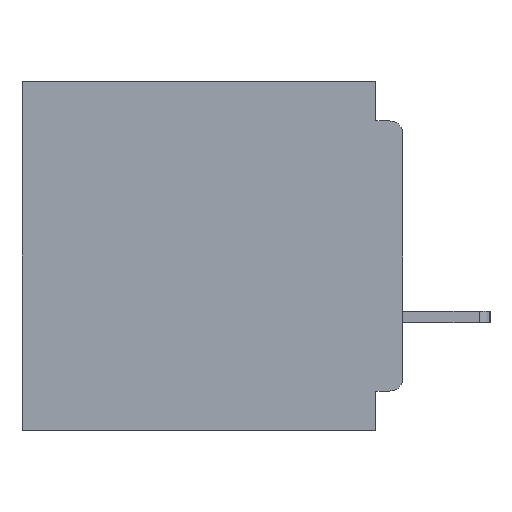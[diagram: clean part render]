
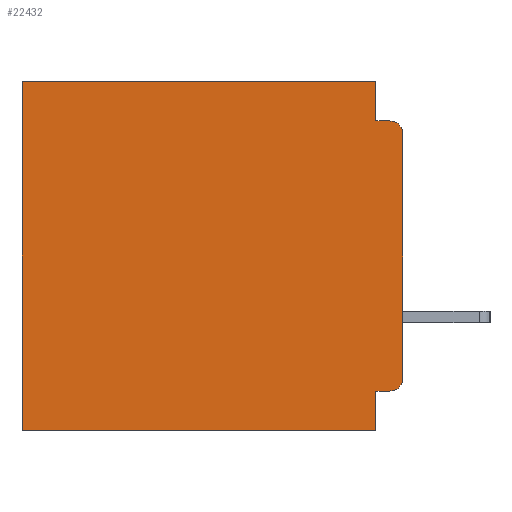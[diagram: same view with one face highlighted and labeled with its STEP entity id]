
A CAD part, left-side view. The second image highlights one B-rep face of the part: STEP entity #22432.
In plain terms, the highlighted planar face has unit normal (-1, 0, 0).
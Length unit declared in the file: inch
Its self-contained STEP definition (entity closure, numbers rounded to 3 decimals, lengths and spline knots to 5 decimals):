
#169 = ORIENTED_EDGE ( 'NONE', *, *, #23646, .F. ) ;
#470 = EDGE_LOOP ( 'NONE', ( #30593, #10990, #30169, #3765, #36550, #21946, #169, #10608, #33827, #23842 ) ) ;
#1314 = CARTESIAN_POINT ( 'NONE',  ( 0.3, 0.437, -0.4 ) ) ;
#1453 = VECTOR ( 'NONE', #3427, 39.37008 ) ;
#2436 = LINE ( 'NONE', #28248, #32483 ) ;
#2808 = DIRECTION ( 'NONE',  ( -1., 0., 0. ) ) ;
#3421 = VERTEX_POINT ( 'NONE', #35032 ) ;
#3427 = DIRECTION ( 'NONE',  ( 0., 0., -1. ) ) ;
#3627 = VERTEX_POINT ( 'NONE', #26118 ) ;
#3765 = ORIENTED_EDGE ( 'NONE', *, *, #23575, .F. ) ;
#4363 = VERTEX_POINT ( 'NONE', #7666 ) ;
#4952 = VERTEX_POINT ( 'NONE', #22074 ) ;
#4992 = DIRECTION ( 'NONE',  ( 0., 0., -1. ) ) ;
#5942 = DIRECTION ( 'NONE',  ( 0., 0., -1. ) ) ;
#5996 = DIRECTION ( 'NONE',  ( 0., 1., 0. ) ) ;
#6307 = VECTOR ( 'NONE', #5942, 39.37008 ) ;
#6898 = VERTEX_POINT ( 'NONE', #21006 ) ;
#7435 = EDGE_CURVE ( 'NONE', #3421, #3627, #36376, .T. ) ;
#7666 = CARTESIAN_POINT ( 'NONE',  ( 0.3, 0.031, -0.4 ) ) ;
#8458 = CIRCLE ( 'NONE', #8766, 0.015 ) ;
#8729 = CARTESIAN_POINT ( 'NONE',  ( 0.3, 0., -0.4 ) ) ;
#8766 = AXIS2_PLACEMENT_3D ( 'NONE', #20181, #2808, #23174 ) ;
#10187 = EDGE_CURVE ( 'NONE', #25279, #13175, #31366, .T. ) ;
#10572 = CARTESIAN_POINT ( 'NONE',  ( 0.3, 0.437, 0. ) ) ;
#10608 = ORIENTED_EDGE ( 'NONE', *, *, #18930, .F. ) ;
#10990 = ORIENTED_EDGE ( 'NONE', *, *, #14570, .T. ) ;
#11297 = CARTESIAN_POINT ( 'NONE',  ( 0.3, 0.031, -0.045 ) ) ;
#11483 = VECTOR ( 'NONE', #22999, 39.37008 ) ;
#11809 = DIRECTION ( 'NONE',  ( 0., 1., 0. ) ) ;
#12071 = EDGE_CURVE ( 'NONE', #3421, #16164, #8458, .T. ) ;
#12117 = DIRECTION ( 'NONE',  ( 1., 0., 0. ) ) ;
#13175 = VERTEX_POINT ( 'NONE', #1314 ) ;
#13344 = EDGE_CURVE ( 'NONE', #25405, #4952, #2436, .T. ) ;
#14570 = EDGE_CURVE ( 'NONE', #19447, #4952, #28294, .T. ) ;
#14644 = AXIS2_PLACEMENT_3D ( 'NONE', #17168, #37584, #20077 ) ;
#15597 = VECTOR ( 'NONE', #31936, 39.37008 ) ;
#15735 = AXIS2_PLACEMENT_3D ( 'NONE', #29598, #12117, #32507 ) ;
#16164 = VERTEX_POINT ( 'NONE', #19823 ) ;
#16492 = LINE ( 'NONE', #34873, #15597 ) ;
#16630 = DIRECTION ( 'NONE',  ( 0., -1., 0. ) ) ;
#17168 = CARTESIAN_POINT ( 'NONE',  ( 0.3, 0.015, -0.06 ) ) ;
#17323 = CARTESIAN_POINT ( 'NONE',  ( 0.3, 0., -0.06 ) ) ;
#18930 = EDGE_CURVE ( 'NONE', #3627, #4363, #31458, .T. ) ;
#19447 = VERTEX_POINT ( 'NONE', #17323 ) ;
#19747 = FACE_OUTER_BOUND ( 'NONE', #470, .T. ) ;
#19823 = CARTESIAN_POINT ( 'NONE',  ( 0.3, 0., -0.34 ) ) ;
#20077 = DIRECTION ( 'NONE',  ( 0., 0., -1. ) ) ;
#20181 = CARTESIAN_POINT ( 'NONE',  ( 0.3, 0.015, -0.34 ) ) ;
#20797 = LINE ( 'NONE', #8729, #6307 ) ;
#20809 = CARTESIAN_POINT ( 'NONE',  ( 0.3, 0.031, -0.4 ) ) ;
#21006 = CARTESIAN_POINT ( 'NONE',  ( 0.3, 0.031, 0. ) ) ;
#21759 = VECTOR ( 'NONE', #11809, 39.37008 ) ;
#21946 = ORIENTED_EDGE ( 'NONE', *, *, #10187, .T. ) ;
#22074 = CARTESIAN_POINT ( 'NONE',  ( 0.3, 0.015, -0.045 ) ) ;
#22432 = ADVANCED_FACE ( 'NONE', ( #19747 ), #23743, .F. ) ;
#22999 = DIRECTION ( 'NONE',  ( 0., 0., -1. ) ) ;
#23174 = DIRECTION ( 'NONE',  ( 0., 0., -1. ) ) ;
#23575 = EDGE_CURVE ( 'NONE', #6898, #25405, #27010, .T. ) ;
#23646 = EDGE_CURVE ( 'NONE', #4363, #13175, #16492, .T. ) ;
#23655 = VECTOR ( 'NONE', #4992, 39.37008 ) ;
#23743 = PLANE ( 'NONE',  #15735 ) ;
#23842 = ORIENTED_EDGE ( 'NONE', *, *, #12071, .T. ) ;
#24206 = VECTOR ( 'NONE', #5996, 39.37008 ) ;
#25102 = LINE ( 'NONE', #29264, #24206 ) ;
#25279 = VERTEX_POINT ( 'NONE', #10572 ) ;
#25405 = VERTEX_POINT ( 'NONE', #11297 ) ;
#26118 = CARTESIAN_POINT ( 'NONE',  ( 0.3, 0.031, -0.355 ) ) ;
#26365 = CARTESIAN_POINT ( 'NONE',  ( 0.3, 0., -0.355 ) ) ;
#27010 = LINE ( 'NONE', #34601, #11483 ) ;
#27103 = EDGE_CURVE ( 'NONE', #19447, #16164, #20797, .T. ) ;
#28248 = CARTESIAN_POINT ( 'NONE',  ( 0.3, 0., -0.045 ) ) ;
#28294 = CIRCLE ( 'NONE', #14644, 0.015 ) ;
#29264 = CARTESIAN_POINT ( 'NONE',  ( 0.3, 0., 0. ) ) ;
#29598 = CARTESIAN_POINT ( 'NONE',  ( 0.3, 0., -0.4 ) ) ;
#30169 = ORIENTED_EDGE ( 'NONE', *, *, #13344, .F. ) ;
#30593 = ORIENTED_EDGE ( 'NONE', *, *, #27103, .F. ) ;
#31036 = EDGE_CURVE ( 'NONE', #6898, #25279, #25102, .T. ) ;
#31366 = LINE ( 'NONE', #36924, #23655 ) ;
#31458 = LINE ( 'NONE', #20809, #1453 ) ;
#31936 = DIRECTION ( 'NONE',  ( 0., 1., 0. ) ) ;
#32483 = VECTOR ( 'NONE', #16630, 39.37008 ) ;
#32507 = DIRECTION ( 'NONE',  ( 0., 0., -1. ) ) ;
#33827 = ORIENTED_EDGE ( 'NONE', *, *, #7435, .F. ) ;
#34601 = CARTESIAN_POINT ( 'NONE',  ( 0.3, 0.031, 0. ) ) ;
#34873 = CARTESIAN_POINT ( 'NONE',  ( 0.3, 0., -0.4 ) ) ;
#35032 = CARTESIAN_POINT ( 'NONE',  ( 0.3, 0.015, -0.355 ) ) ;
#36376 = LINE ( 'NONE', #26365, #21759 ) ;
#36550 = ORIENTED_EDGE ( 'NONE', *, *, #31036, .T. ) ;
#36924 = CARTESIAN_POINT ( 'NONE',  ( 0.3, 0.437, -0.4 ) ) ;
#37584 = DIRECTION ( 'NONE',  ( -1., 0., 0. ) ) ;
